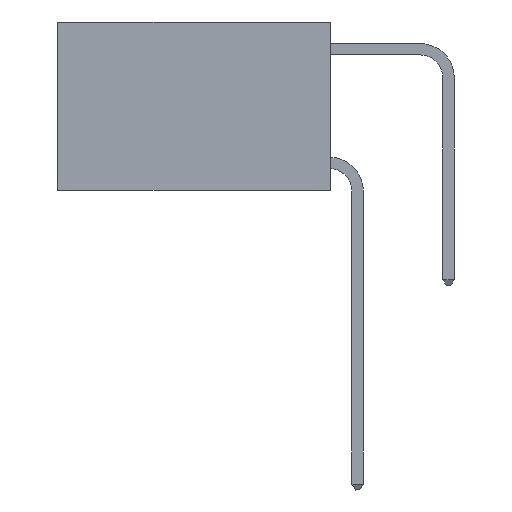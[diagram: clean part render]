
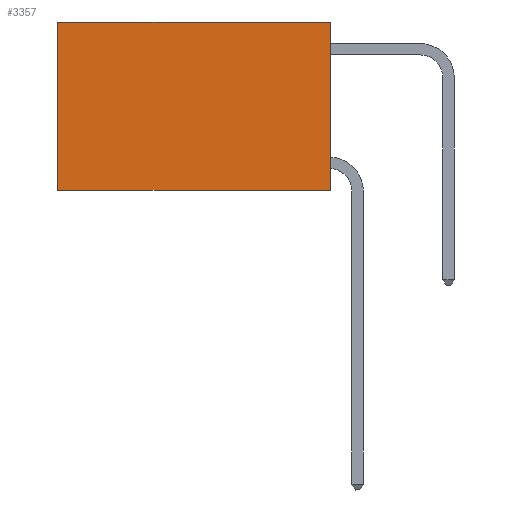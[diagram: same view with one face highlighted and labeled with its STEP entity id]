
A CAD part, left-side view. The second image highlights one B-rep face of the part: STEP entity #3357.
In plain terms, the highlighted planar face has unit normal (-1, 0, 0).
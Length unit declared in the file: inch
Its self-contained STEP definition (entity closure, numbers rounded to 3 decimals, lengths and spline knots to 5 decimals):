
#446 = CARTESIAN_POINT ( 'NONE',  ( 0.2625, 0., 0. ) ) ;
#646 = VERTEX_POINT ( 'NONE', #4172 ) ;
#790 = EDGE_CURVE ( 'NONE', #2531, #7648, #5654, .T. ) ;
#1141 = DIRECTION ( 'NONE',  ( 0., 1., 0. ) ) ;
#1588 = VECTOR ( 'NONE', #2678, 39.37008 ) ;
#1618 = CARTESIAN_POINT ( 'NONE',  ( 0.2625, 0., -0.37 ) ) ;
#1620 = LINE ( 'NONE', #2728, #1588 ) ;
#1702 = DIRECTION ( 'NONE',  ( 0., 1., 0. ) ) ;
#2095 = VECTOR ( 'NONE', #1702, 39.37008 ) ;
#2176 = EDGE_CURVE ( 'NONE', #646, #7648, #3018, .T. ) ;
#2531 = VERTEX_POINT ( 'NONE', #4850 ) ;
#2678 = DIRECTION ( 'NONE',  ( 0., 0., -1. ) ) ;
#2728 = CARTESIAN_POINT ( 'NONE',  ( 0.2625, 0., 0. ) ) ;
#2792 = DIRECTION ( 'NONE',  ( 0., 0., -1. ) ) ;
#3018 = LINE ( 'NONE', #1618, #2095 ) ;
#3263 = CARTESIAN_POINT ( 'NONE',  ( 0.2625, 0.6, 0. ) ) ;
#3357 = ADVANCED_FACE ( 'NONE', ( #6200 ), #6185, .F. ) ;
#3676 = VECTOR ( 'NONE', #1141, 39.37008 ) ;
#3723 = EDGE_CURVE ( 'NONE', #4054, #646, #1620, .T. ) ;
#4054 = VERTEX_POINT ( 'NONE', #446 ) ;
#4172 = CARTESIAN_POINT ( 'NONE',  ( 0.2625, 0., -0.37 ) ) ;
#4850 = CARTESIAN_POINT ( 'NONE',  ( 0.2625, 0.6, 0. ) ) ;
#5434 = CARTESIAN_POINT ( 'NONE',  ( 0.2625, 0., 0. ) ) ;
#5654 = LINE ( 'NONE', #3263, #6501 ) ;
#5655 = ORIENTED_EDGE ( 'NONE', *, *, #790, .T. ) ;
#6117 = DIRECTION ( 'NONE',  ( 0., 0., -1. ) ) ;
#6157 = DIRECTION ( 'NONE',  ( 1., 0., 0. ) ) ;
#6185 = PLANE ( 'NONE',  #7697 ) ;
#6200 = FACE_OUTER_BOUND ( 'NONE', #9082, .T. ) ;
#6201 = CARTESIAN_POINT ( 'NONE',  ( 0.2625, 0., 0. ) ) ;
#6501 = VECTOR ( 'NONE', #2792, 39.37008 ) ;
#6603 = LINE ( 'NONE', #5434, #3676 ) ;
#6825 = ORIENTED_EDGE ( 'NONE', *, *, #10175, .T. ) ;
#7308 = ORIENTED_EDGE ( 'NONE', *, *, #2176, .F. ) ;
#7361 = ORIENTED_EDGE ( 'NONE', *, *, #3723, .F. ) ;
#7377 = CARTESIAN_POINT ( 'NONE',  ( 0.2625, 0.6, -0.37 ) ) ;
#7648 = VERTEX_POINT ( 'NONE', #7377 ) ;
#7697 = AXIS2_PLACEMENT_3D ( 'NONE', #6201, #6157, #6117 ) ;
#9082 = EDGE_LOOP ( 'NONE', ( #5655, #7308, #7361, #6825 ) ) ;
#10175 = EDGE_CURVE ( 'NONE', #4054, #2531, #6603, .T. ) ;
